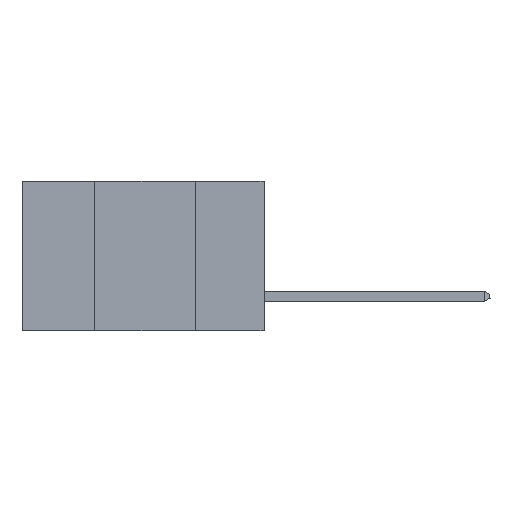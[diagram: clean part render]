
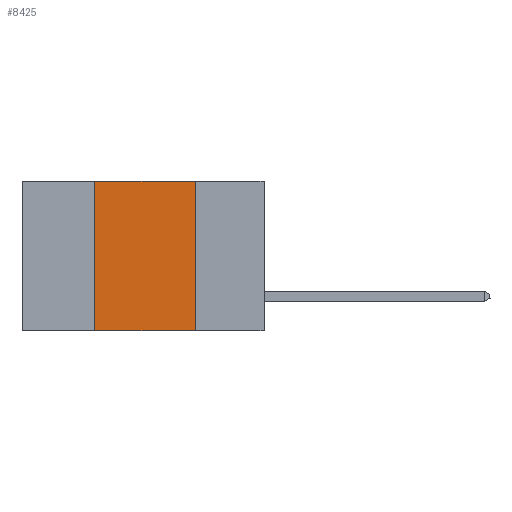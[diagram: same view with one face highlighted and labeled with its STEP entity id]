
A CAD part, left-side view. The second image highlights one B-rep face of the part: STEP entity #8425.
In plain terms, the highlighted planar face has unit normal (-1, 0, 0).
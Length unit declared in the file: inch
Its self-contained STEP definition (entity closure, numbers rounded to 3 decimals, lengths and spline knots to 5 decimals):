
#347 = CARTESIAN_POINT ( 'NONE',  ( 0., 0.6, 0. ) ) ;
#411 = DIRECTION ( 'NONE',  ( 0., 0., -1. ) ) ;
#728 = AXIS2_PLACEMENT_3D ( 'NONE', #347, #7974, #411 ) ;
#772 = CARTESIAN_POINT ( 'NONE',  ( 0., 0.17, -0.37 ) ) ;
#1230 = VECTOR ( 'NONE', #8763, 39.37008 ) ;
#1304 = EDGE_CURVE ( 'NONE', #9619, #3483, #2227, .T. ) ;
#1386 = VECTOR ( 'NONE', #1829, 39.37008 ) ;
#1424 = LINE ( 'NONE', #5701, #9311 ) ;
#1829 = DIRECTION ( 'NONE',  ( 0., -1., 0. ) ) ;
#1842 = PLANE ( 'NONE',  #728 ) ;
#2227 = LINE ( 'NONE', #4219, #1386 ) ;
#3147 = ORIENTED_EDGE ( 'NONE', *, *, #8450, .F. ) ;
#3483 = VERTEX_POINT ( 'NONE', #6374 ) ;
#3495 = CARTESIAN_POINT ( 'NONE',  ( 0., 0.6, -0.37 ) ) ;
#3939 = ORIENTED_EDGE ( 'NONE', *, *, #6859, .T. ) ;
#4219 = CARTESIAN_POINT ( 'NONE',  ( 0., 0.6, 0. ) ) ;
#4631 = CARTESIAN_POINT ( 'NONE',  ( 0., 0.17, 0. ) ) ;
#4726 = LINE ( 'NONE', #3495, #1230 ) ;
#4812 = VERTEX_POINT ( 'NONE', #6485 ) ;
#5301 = VECTOR ( 'NONE', #9344, 39.37008 ) ;
#5701 = CARTESIAN_POINT ( 'NONE',  ( 0., 0.42, 0. ) ) ;
#6209 = VERTEX_POINT ( 'NONE', #772 ) ;
#6374 = CARTESIAN_POINT ( 'NONE',  ( 0., 0.17, 0. ) ) ;
#6485 = CARTESIAN_POINT ( 'NONE',  ( 0., 0.42, -0.37 ) ) ;
#6486 = DIRECTION ( 'NONE',  ( 0., 0., 1. ) ) ;
#6859 = EDGE_CURVE ( 'NONE', #4812, #6209, #4726, .T. ) ;
#6958 = LINE ( 'NONE', #4631, #5301 ) ;
#7974 = DIRECTION ( 'NONE',  ( 1., 0., 0. ) ) ;
#8425 = ADVANCED_FACE ( 'NONE', ( #8834 ), #1842, .F. ) ;
#8450 = EDGE_CURVE ( 'NONE', #4812, #9619, #1424, .T. ) ;
#8478 = EDGE_LOOP ( 'NONE', ( #8949, #8481, #3147, #3939 ) ) ;
#8481 = ORIENTED_EDGE ( 'NONE', *, *, #1304, .F. ) ;
#8763 = DIRECTION ( 'NONE',  ( 0., -1., 0. ) ) ;
#8834 = FACE_OUTER_BOUND ( 'NONE', #8478, .T. ) ;
#8949 = ORIENTED_EDGE ( 'NONE', *, *, #9102, .F. ) ;
#8975 = CARTESIAN_POINT ( 'NONE',  ( 0., 0.42, 0. ) ) ;
#9102 = EDGE_CURVE ( 'NONE', #3483, #6209, #6958, .T. ) ;
#9311 = VECTOR ( 'NONE', #6486, 39.37008 ) ;
#9344 = DIRECTION ( 'NONE',  ( 0., 0., -1. ) ) ;
#9619 = VERTEX_POINT ( 'NONE', #8975 ) ;
